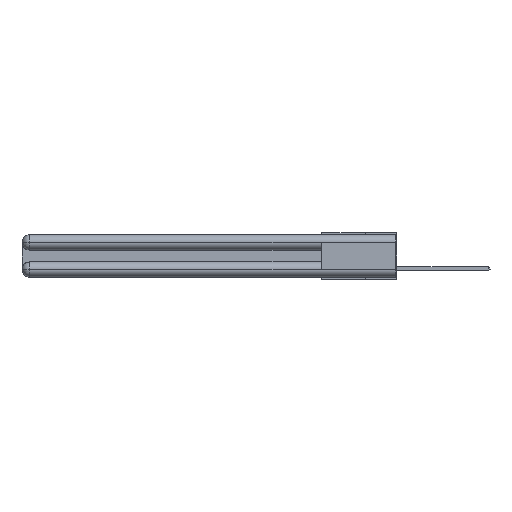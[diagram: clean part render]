
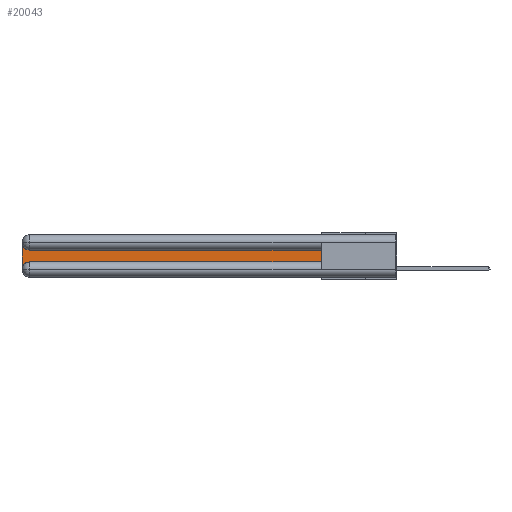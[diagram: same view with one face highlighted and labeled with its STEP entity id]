
A CAD part, left-side view. The second image highlights one B-rep face of the part: STEP entity #20043.
In plain terms, the highlighted planar face has unit normal (-1, 0, 0).
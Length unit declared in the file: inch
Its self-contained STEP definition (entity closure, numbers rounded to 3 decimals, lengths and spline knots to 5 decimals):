
#309 = CARTESIAN_POINT ( 'NONE',  ( 0.075, 3., -0.2175 ) ) ;
#2066 = ORIENTED_EDGE ( 'NONE', *, *, #10236, .T. ) ;
#3179 = DIRECTION ( 'NONE',  ( 0., 0., -1. ) ) ;
#4147 = VERTEX_POINT ( 'NONE', #13930 ) ;
#4416 = CARTESIAN_POINT ( 'NONE',  ( 0.075, 3., -0.1225 ) ) ;
#4821 = VERTEX_POINT ( 'NONE', #19510 ) ;
#5221 = VERTEX_POINT ( 'NONE', #15033 ) ;
#5295 = AXIS2_PLACEMENT_3D ( 'NONE', #9131, #13607, #18678 ) ;
#8194 = CARTESIAN_POINT ( 'NONE',  ( 0.075, 3., -0.0625 ) ) ;
#8582 = CIRCLE ( 'NONE', #5295, 0.06 ) ;
#9131 = CARTESIAN_POINT ( 'NONE',  ( 0.075, 2.94, -0.2775 ) ) ;
#9348 = LINE ( 'NONE', #309, #23168 ) ;
#10236 = EDGE_CURVE ( 'NONE', #24304, #18002, #9348, .T. ) ;
#10351 = EDGE_CURVE ( 'NONE', #18002, #4821, #8582, .T. ) ;
#10701 = LINE ( 'NONE', #14317, #25689 ) ;
#13607 = DIRECTION ( 'NONE',  ( 1., 0., 0. ) ) ;
#13614 = CARTESIAN_POINT ( 'NONE',  ( 0.075, 0.6, -0.2175 ) ) ;
#13757 = CARTESIAN_POINT ( 'NONE',  ( 0.075, 3., -0.2775 ) ) ;
#13930 = CARTESIAN_POINT ( 'NONE',  ( 0.075, 0.6, -0.1225 ) ) ;
#14206 = DIRECTION ( 'NONE',  ( 0., -1., 0. ) ) ;
#14317 = CARTESIAN_POINT ( 'NONE',  ( 0.075, 0.6, -0.2175 ) ) ;
#14835 = CARTESIAN_POINT ( 'NONE',  ( 0.075, 0.6, -0.1225 ) ) ;
#14935 = AXIS2_PLACEMENT_3D ( 'NONE', #4416, #26760, #24208 ) ;
#15033 = CARTESIAN_POINT ( 'NONE',  ( 0.075, 0.6, -0.2175 ) ) ;
#15134 = LINE ( 'NONE', #13614, #31648 ) ;
#15249 = FACE_OUTER_BOUND ( 'NONE', #26061, .T. ) ;
#16796 = DIRECTION ( 'NONE',  ( 0., 0., -1. ) ) ;
#17149 = VERTEX_POINT ( 'NONE', #26799 ) ;
#17217 = DIRECTION ( 'NONE',  ( 0., 1., 0. ) ) ;
#18002 = VERTEX_POINT ( 'NONE', #13757 ) ;
#18583 = DIRECTION ( 'NONE',  ( 0., 0., 1. ) ) ;
#18678 = DIRECTION ( 'NONE',  ( 0., 0., -1. ) ) ;
#19280 = CIRCLE ( 'NONE', #22897, 0.06 ) ;
#19361 = EDGE_CURVE ( 'NONE', #4821, #5221, #10701, .T. ) ;
#19510 = CARTESIAN_POINT ( 'NONE',  ( 0.075, 2.94, -0.2175 ) ) ;
#19867 = ORIENTED_EDGE ( 'NONE', *, *, #21240, .T. ) ;
#20043 = ADVANCED_FACE ( 'NONE', ( #15249 ), #31202, .F. ) ;
#21240 = EDGE_CURVE ( 'NONE', #5221, #4147, #15134, .T. ) ;
#22603 = ORIENTED_EDGE ( 'NONE', *, *, #19361, .T. ) ;
#22897 = AXIS2_PLACEMENT_3D ( 'NONE', #24035, #31226, #16796 ) ;
#23168 = VECTOR ( 'NONE', #3179, 39.37008 ) ;
#24035 = CARTESIAN_POINT ( 'NONE',  ( 0.075, 2.94, -0.0625 ) ) ;
#24208 = DIRECTION ( 'NONE',  ( 0., 0., -1. ) ) ;
#24304 = VERTEX_POINT ( 'NONE', #8194 ) ;
#25051 = VECTOR ( 'NONE', #17217, 39.37008 ) ;
#25689 = VECTOR ( 'NONE', #14206, 39.37008 ) ;
#26061 = EDGE_LOOP ( 'NONE', ( #27428, #28239, #2066, #30133, #22603, #19867 ) ) ;
#26524 = EDGE_CURVE ( 'NONE', #4147, #17149, #31548, .T. ) ;
#26760 = DIRECTION ( 'NONE',  ( 1., 0., 0. ) ) ;
#26799 = CARTESIAN_POINT ( 'NONE',  ( 0.075, 2.94, -0.1225 ) ) ;
#27428 = ORIENTED_EDGE ( 'NONE', *, *, #26524, .T. ) ;
#28239 = ORIENTED_EDGE ( 'NONE', *, *, #31267, .T. ) ;
#30133 = ORIENTED_EDGE ( 'NONE', *, *, #10351, .T. ) ;
#31202 = PLANE ( 'NONE',  #14935 ) ;
#31226 = DIRECTION ( 'NONE',  ( 1., 0., 0. ) ) ;
#31267 = EDGE_CURVE ( 'NONE', #17149, #24304, #19280, .T. ) ;
#31548 = LINE ( 'NONE', #14835, #25051 ) ;
#31648 = VECTOR ( 'NONE', #18583, 39.37008 ) ;
